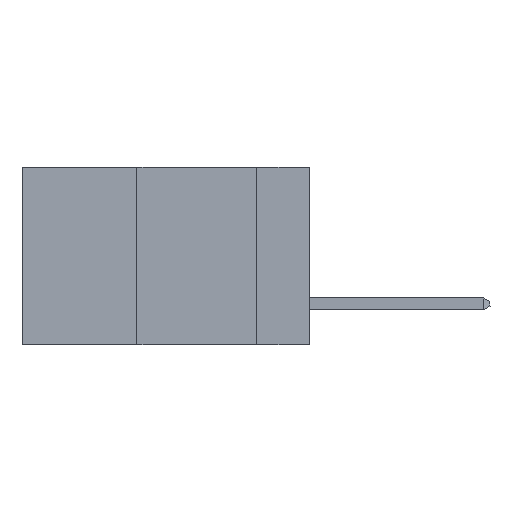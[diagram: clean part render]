
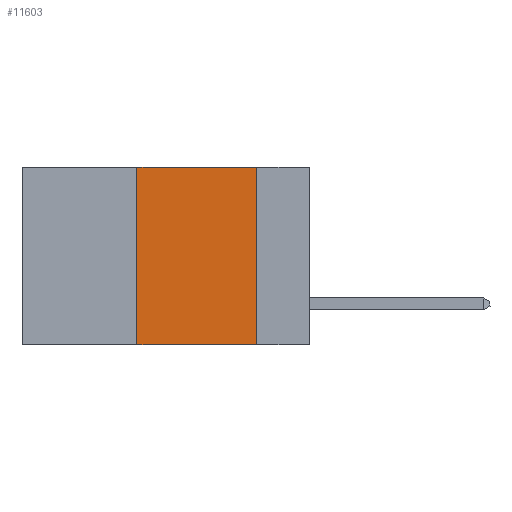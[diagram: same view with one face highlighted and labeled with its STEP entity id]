
A CAD part, left-side view. The second image highlights one B-rep face of the part: STEP entity #11603.
In plain terms, the highlighted planar face has unit normal (-1, 0, 0).
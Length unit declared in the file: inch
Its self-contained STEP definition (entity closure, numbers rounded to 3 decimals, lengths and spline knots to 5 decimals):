
#1119 = PLANE ( 'NONE',  #5327 ) ;
#1188 = CARTESIAN_POINT ( 'NONE',  ( 0., 0.11, 0. ) ) ;
#1472 = VERTEX_POINT ( 'NONE', #17740 ) ;
#1550 = EDGE_LOOP ( 'NONE', ( #18719, #19088, #1720, #18674 ) ) ;
#1720 = ORIENTED_EDGE ( 'NONE', *, *, #12334, .F. ) ;
#3288 = CARTESIAN_POINT ( 'NONE',  ( 0., 0.36, -0.37 ) ) ;
#4724 = DIRECTION ( 'NONE',  ( 1., 0., 0. ) ) ;
#4976 = EDGE_CURVE ( 'NONE', #7620, #12854, #13213, .T. ) ;
#5327 = AXIS2_PLACEMENT_3D ( 'NONE', #15618, #4724, #17406 ) ;
#5558 = CARTESIAN_POINT ( 'NONE',  ( 0., 0.6, 0. ) ) ;
#5815 = CARTESIAN_POINT ( 'NONE',  ( 0., 0.11, 0. ) ) ;
#7238 = DIRECTION ( 'NONE',  ( 0., 0., 1. ) ) ;
#7620 = VERTEX_POINT ( 'NONE', #3288 ) ;
#9463 = DIRECTION ( 'NONE',  ( 0., 0., -1. ) ) ;
#9767 = VERTEX_POINT ( 'NONE', #1188 ) ;
#10902 = VECTOR ( 'NONE', #9463, 39.37008 ) ;
#10941 = CARTESIAN_POINT ( 'NONE',  ( 0., 0.36, 0. ) ) ;
#10975 = FACE_OUTER_BOUND ( 'NONE', #1550, .T. ) ;
#11603 = ADVANCED_FACE ( 'NONE', ( #10975 ), #1119, .F. ) ;
#11803 = LINE ( 'NONE', #5558, #16592 ) ;
#12334 = EDGE_CURVE ( 'NONE', #7620, #1472, #17951, .T. ) ;
#12376 = CARTESIAN_POINT ( 'NONE',  ( 0., 0.11, -0.37 ) ) ;
#12627 = VECTOR ( 'NONE', #19789, 39.37008 ) ;
#12854 = VERTEX_POINT ( 'NONE', #12376 ) ;
#13213 = LINE ( 'NONE', #19744, #12627 ) ;
#15618 = CARTESIAN_POINT ( 'NONE',  ( 0., 0.6, 0. ) ) ;
#16592 = VECTOR ( 'NONE', #19951, 39.37008 ) ;
#17406 = DIRECTION ( 'NONE',  ( 0., 0., -1. ) ) ;
#17740 = CARTESIAN_POINT ( 'NONE',  ( 0., 0.36, 0. ) ) ;
#17951 = LINE ( 'NONE', #10941, #19058 ) ;
#18157 = EDGE_CURVE ( 'NONE', #1472, #9767, #11803, .T. ) ;
#18674 = ORIENTED_EDGE ( 'NONE', *, *, #4976, .T. ) ;
#18719 = ORIENTED_EDGE ( 'NONE', *, *, #19468, .F. ) ;
#19058 = VECTOR ( 'NONE', #7238, 39.37008 ) ;
#19088 = ORIENTED_EDGE ( 'NONE', *, *, #18157, .F. ) ;
#19468 = EDGE_CURVE ( 'NONE', #9767, #12854, #20356, .T. ) ;
#19744 = CARTESIAN_POINT ( 'NONE',  ( 0., 0.6, -0.37 ) ) ;
#19789 = DIRECTION ( 'NONE',  ( 0., -1., 0. ) ) ;
#19951 = DIRECTION ( 'NONE',  ( 0., -1., 0. ) ) ;
#20356 = LINE ( 'NONE', #5815, #10902 ) ;
